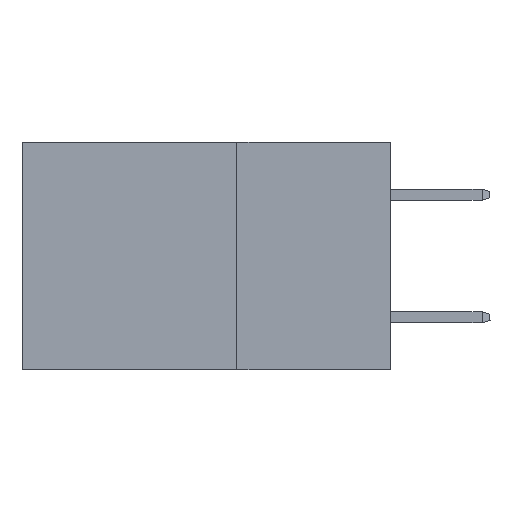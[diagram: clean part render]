
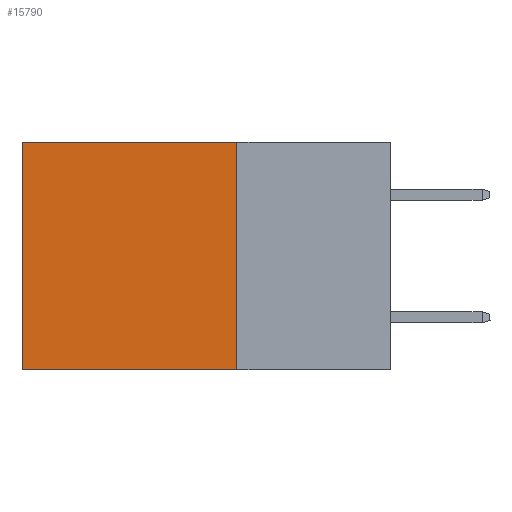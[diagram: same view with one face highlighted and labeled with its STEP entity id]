
A CAD part, left-side view. The second image highlights one B-rep face of the part: STEP entity #15790.
In plain terms, the highlighted planar face has unit normal (-1, 0, 0).
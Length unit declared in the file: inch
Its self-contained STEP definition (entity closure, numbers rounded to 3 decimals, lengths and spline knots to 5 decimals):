
#811 = DIRECTION ( 'NONE',  ( 0., 1., 0. ) ) ;
#1402 = CARTESIAN_POINT ( 'NONE',  ( 0.2875, 0.6, 0. ) ) ;
#2191 = LINE ( 'NONE', #11357, #12759 ) ;
#3072 = PLANE ( 'NONE',  #19103 ) ;
#3657 = LINE ( 'NONE', #16532, #19132 ) ;
#4247 = CARTESIAN_POINT ( 'NONE',  ( 0.2875, 0.6, -0.37 ) ) ;
#4812 = VERTEX_POINT ( 'NONE', #4247 ) ;
#4869 = ORIENTED_EDGE ( 'NONE', *, *, #12793, .T. ) ;
#5273 = DIRECTION ( 'NONE',  ( 1., 0., 0. ) ) ;
#5937 = EDGE_CURVE ( 'NONE', #8297, #4812, #7891, .T. ) ;
#6000 = DIRECTION ( 'NONE',  ( 0., 0., -1. ) ) ;
#6075 = FACE_OUTER_BOUND ( 'NONE', #7197, .T. ) ;
#7197 = EDGE_LOOP ( 'NONE', ( #8998, #10295, #10211, #4869 ) ) ;
#7242 = VECTOR ( 'NONE', #14061, 39.37008 ) ;
#7891 = LINE ( 'NONE', #1402, #7242 ) ;
#8297 = VERTEX_POINT ( 'NONE', #24942 ) ;
#8854 = VERTEX_POINT ( 'NONE', #12041 ) ;
#8998 = ORIENTED_EDGE ( 'NONE', *, *, #5937, .T. ) ;
#9779 = CARTESIAN_POINT ( 'NONE',  ( 0.2875, 0.25, 0. ) ) ;
#10211 = ORIENTED_EDGE ( 'NONE', *, *, #17913, .F. ) ;
#10295 = ORIENTED_EDGE ( 'NONE', *, *, #23298, .F. ) ;
#10368 = VERTEX_POINT ( 'NONE', #13722 ) ;
#11357 = CARTESIAN_POINT ( 'NONE',  ( 0.2875, 0.25, -0.37 ) ) ;
#11497 = LINE ( 'NONE', #9779, #21946 ) ;
#11546 = CARTESIAN_POINT ( 'NONE',  ( 0.2875, 0.25, 0. ) ) ;
#12041 = CARTESIAN_POINT ( 'NONE',  ( 0.2875, 0.25, -0.37 ) ) ;
#12759 = VECTOR ( 'NONE', #811, 39.37008 ) ;
#12793 = EDGE_CURVE ( 'NONE', #10368, #8297, #11497, .T. ) ;
#13722 = CARTESIAN_POINT ( 'NONE',  ( 0.2875, 0.25, 0. ) ) ;
#14061 = DIRECTION ( 'NONE',  ( 0., 0., -1. ) ) ;
#15790 = ADVANCED_FACE ( 'NONE', ( #6075 ), #3072, .F. ) ;
#16532 = CARTESIAN_POINT ( 'NONE',  ( 0.2875, 0.25, 0. ) ) ;
#17913 = EDGE_CURVE ( 'NONE', #10368, #8854, #3657, .T. ) ;
#19103 = AXIS2_PLACEMENT_3D ( 'NONE', #11546, #5273, #19978 ) ;
#19132 = VECTOR ( 'NONE', #6000, 39.37008 ) ;
#19978 = DIRECTION ( 'NONE',  ( 0., 0., -1. ) ) ;
#21946 = VECTOR ( 'NONE', #24345, 39.37008 ) ;
#23298 = EDGE_CURVE ( 'NONE', #8854, #4812, #2191, .T. ) ;
#24345 = DIRECTION ( 'NONE',  ( 0., 1., 0. ) ) ;
#24942 = CARTESIAN_POINT ( 'NONE',  ( 0.2875, 0.6, 0. ) ) ;
